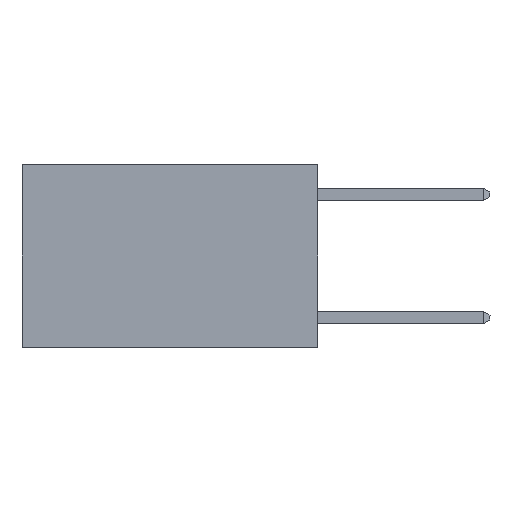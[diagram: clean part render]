
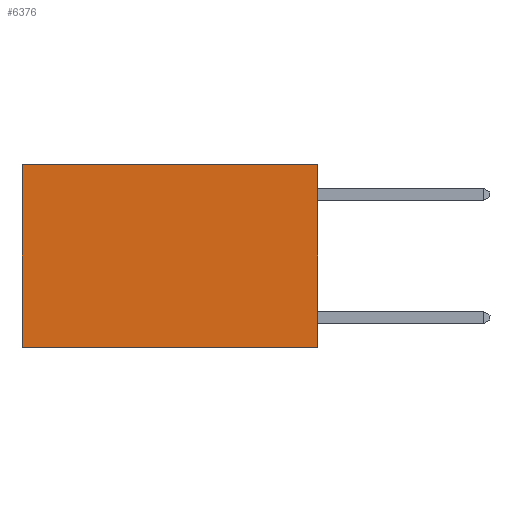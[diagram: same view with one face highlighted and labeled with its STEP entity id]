
A CAD part, left-side view. The second image highlights one B-rep face of the part: STEP entity #6376.
In plain terms, the highlighted planar face has unit normal (-1, 0, 0).
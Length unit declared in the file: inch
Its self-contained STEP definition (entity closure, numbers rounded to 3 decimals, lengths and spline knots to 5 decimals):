
#1095 = VERTEX_POINT ( 'NONE', #2957 ) ;
#1151 = CARTESIAN_POINT ( 'NONE',  ( 0.2625, 0., 0. ) ) ;
#1169 = EDGE_LOOP ( 'NONE', ( #1370, #1633, #4293, #2793 ) ) ;
#1245 = DIRECTION ( 'NONE',  ( 0., 0., -1. ) ) ;
#1255 = EDGE_CURVE ( 'NONE', #2534, #1095, #3497, .T. ) ;
#1370 = ORIENTED_EDGE ( 'NONE', *, *, #5782, .T. ) ;
#1418 = CARTESIAN_POINT ( 'NONE',  ( 0.2625, 0.6, 0. ) ) ;
#1633 = ORIENTED_EDGE ( 'NONE', *, *, #3994, .F. ) ;
#1634 = VECTOR ( 'NONE', #1245, 39.37008 ) ;
#1914 = LINE ( 'NONE', #6734, #6726 ) ;
#2399 = VECTOR ( 'NONE', #3641, 39.37008 ) ;
#2534 = VERTEX_POINT ( 'NONE', #7352 ) ;
#2699 = PLANE ( 'NONE',  #4583 ) ;
#2793 = ORIENTED_EDGE ( 'NONE', *, *, #6375, .T. ) ;
#2957 = CARTESIAN_POINT ( 'NONE',  ( 0.2625, 0., -0.37 ) ) ;
#3006 = VECTOR ( 'NONE', #6178, 39.37008 ) ;
#3497 = LINE ( 'NONE', #1151, #1634 ) ;
#3574 = CARTESIAN_POINT ( 'NONE',  ( 0.2625, 0., -0.37 ) ) ;
#3641 = DIRECTION ( 'NONE',  ( 0., 1., 0. ) ) ;
#3963 = FACE_OUTER_BOUND ( 'NONE', #1169, .T. ) ;
#3994 = EDGE_CURVE ( 'NONE', #1095, #7123, #5995, .T. ) ;
#4088 = CARTESIAN_POINT ( 'NONE',  ( 0.2625, 0., 0. ) ) ;
#4293 = ORIENTED_EDGE ( 'NONE', *, *, #1255, .F. ) ;
#4583 = AXIS2_PLACEMENT_3D ( 'NONE', #4088, #8754, #4761 ) ;
#4761 = DIRECTION ( 'NONE',  ( 0., 0., -1. ) ) ;
#5481 = VERTEX_POINT ( 'NONE', #7065 ) ;
#5782 = EDGE_CURVE ( 'NONE', #5481, #7123, #6371, .T. ) ;
#5995 = LINE ( 'NONE', #3574, #2399 ) ;
#6060 = DIRECTION ( 'NONE',  ( 0., 1., 0. ) ) ;
#6178 = DIRECTION ( 'NONE',  ( 0., 0., -1. ) ) ;
#6371 = LINE ( 'NONE', #1418, #3006 ) ;
#6375 = EDGE_CURVE ( 'NONE', #2534, #5481, #1914, .T. ) ;
#6376 = ADVANCED_FACE ( 'NONE', ( #3963 ), #2699, .F. ) ;
#6726 = VECTOR ( 'NONE', #6060, 39.37008 ) ;
#6734 = CARTESIAN_POINT ( 'NONE',  ( 0.2625, 0., 0. ) ) ;
#7065 = CARTESIAN_POINT ( 'NONE',  ( 0.2625, 0.6, 0. ) ) ;
#7123 = VERTEX_POINT ( 'NONE', #7516 ) ;
#7352 = CARTESIAN_POINT ( 'NONE',  ( 0.2625, 0., 0. ) ) ;
#7516 = CARTESIAN_POINT ( 'NONE',  ( 0.2625, 0.6, -0.37 ) ) ;
#8754 = DIRECTION ( 'NONE',  ( 1., 0., 0. ) ) ;
